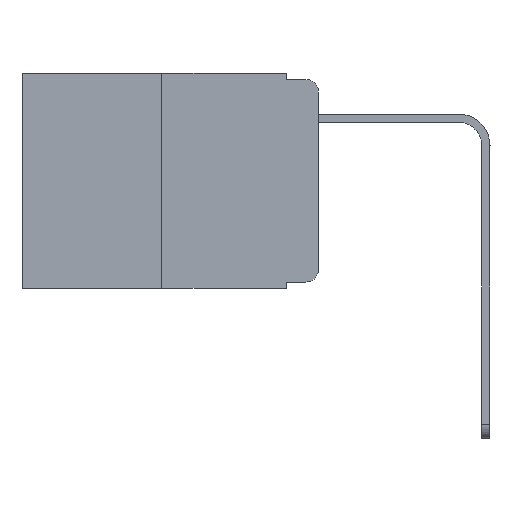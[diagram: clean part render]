
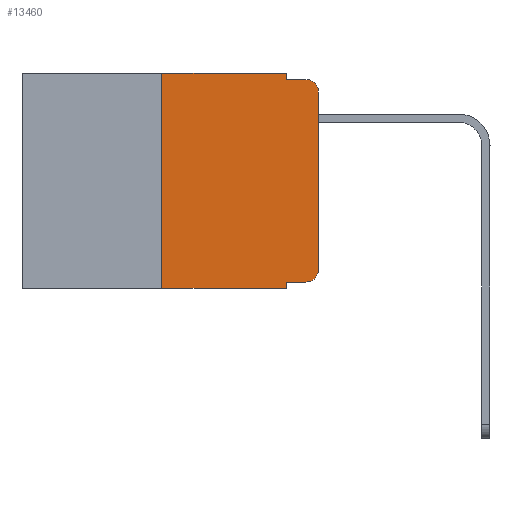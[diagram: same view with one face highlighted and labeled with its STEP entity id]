
A CAD part, left-side view. The second image highlights one B-rep face of the part: STEP entity #13460.
In plain terms, the highlighted planar face has unit normal (-1, 0, 0).
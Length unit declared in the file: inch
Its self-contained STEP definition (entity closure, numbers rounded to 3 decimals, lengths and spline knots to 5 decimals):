
#66 = ORIENTED_EDGE ( 'NONE', *, *, #15885, .T. ) ;
#69 = DIRECTION ( 'NONE',  ( 0., 0., -1. ) ) ;
#484 = CARTESIAN_POINT ( 'NONE',  ( 0., 0.051, -0.333 ) ) ;
#685 = CARTESIAN_POINT ( 'NONE',  ( 0., 0.02, -0.313 ) ) ;
#712 = CARTESIAN_POINT ( 'NONE',  ( 0., 0.473, 0. ) ) ;
#753 = VERTEX_POINT ( 'NONE', #1145 ) ;
#788 = CARTESIAN_POINT ( 'NONE',  ( 0., 0.02, -0.333 ) ) ;
#983 = AXIS2_PLACEMENT_3D ( 'NONE', #712, #11700, #2140 ) ;
#1099 = VERTEX_POINT ( 'NONE', #9151 ) ;
#1145 = CARTESIAN_POINT ( 'NONE',  ( 0., 0.051, 0. ) ) ;
#1576 = CARTESIAN_POINT ( 'NONE',  ( 0., 0.25, 0. ) ) ;
#1659 = CARTESIAN_POINT ( 'NONE',  ( 0., 0., -0.313 ) ) ;
#1747 = CARTESIAN_POINT ( 'NONE',  ( 0., 0.051, -0.01 ) ) ;
#1787 = CARTESIAN_POINT ( 'NONE',  ( 0., 0.473, -0.343 ) ) ;
#2140 = DIRECTION ( 'NONE',  ( 0., 0., -1. ) ) ;
#2186 = AXIS2_PLACEMENT_3D ( 'NONE', #685, #13418, #4994 ) ;
#2284 = ORIENTED_EDGE ( 'NONE', *, *, #7807, .F. ) ;
#2453 = VERTEX_POINT ( 'NONE', #1747 ) ;
#2645 = ORIENTED_EDGE ( 'NONE', *, *, #8394, .T. ) ;
#2680 = EDGE_CURVE ( 'NONE', #7427, #15474, #4376, .T. ) ;
#2983 = FACE_OUTER_BOUND ( 'NONE', #12469, .T. ) ;
#3580 = LINE ( 'NONE', #10822, #18109 ) ;
#3884 = CARTESIAN_POINT ( 'NONE',  ( 0., 0.051, -0.01 ) ) ;
#3978 = VERTEX_POINT ( 'NONE', #9207 ) ;
#4061 = CARTESIAN_POINT ( 'NONE',  ( 0., 0.02, -0.01 ) ) ;
#4107 = VECTOR ( 'NONE', #14546, 39.37008 ) ;
#4376 = CIRCLE ( 'NONE', #2186, 0.02 ) ;
#4994 = DIRECTION ( 'NONE',  ( 0., 0., -1. ) ) ;
#5096 = EDGE_CURVE ( 'NONE', #13319, #7427, #9376, .T. ) ;
#5805 = CARTESIAN_POINT ( 'NONE',  ( 0., 0.051, -0.333 ) ) ;
#6109 = EDGE_CURVE ( 'NONE', #753, #2453, #14809, .T. ) ;
#6309 = ORIENTED_EDGE ( 'NONE', *, *, #13696, .T. ) ;
#6413 = VERTEX_POINT ( 'NONE', #13364 ) ;
#6456 = ORIENTED_EDGE ( 'NONE', *, *, #7017, .F. ) ;
#6510 = CARTESIAN_POINT ( 'NONE',  ( 0., 0.02, -0.03 ) ) ;
#7017 = EDGE_CURVE ( 'NONE', #2453, #7630, #15676, .T. ) ;
#7042 = EDGE_CURVE ( 'NONE', #3978, #753, #3580, .T. ) ;
#7072 = CARTESIAN_POINT ( 'NONE',  ( 0., 0.051, 0. ) ) ;
#7427 = VERTEX_POINT ( 'NONE', #788 ) ;
#7570 = VECTOR ( 'NONE', #11715, 39.37008 ) ;
#7630 = VERTEX_POINT ( 'NONE', #4061 ) ;
#7807 = EDGE_CURVE ( 'NONE', #1099, #3978, #15631, .T. ) ;
#7933 = DIRECTION ( 'NONE',  ( 0., 0., -1. ) ) ;
#8123 = DIRECTION ( 'NONE',  ( 0., -1., 0. ) ) ;
#8161 = CARTESIAN_POINT ( 'NONE',  ( 0., 0., 0. ) ) ;
#8382 = VECTOR ( 'NONE', #17199, 39.37008 ) ;
#8394 = EDGE_CURVE ( 'NONE', #1099, #17314, #15501, .T. ) ;
#8700 = VECTOR ( 'NONE', #13808, 39.37008 ) ;
#9151 = CARTESIAN_POINT ( 'NONE',  ( 0., 0.25, -0.343 ) ) ;
#9207 = CARTESIAN_POINT ( 'NONE',  ( 0., 0.25, 0. ) ) ;
#9376 = LINE ( 'NONE', #484, #4107 ) ;
#9874 = CIRCLE ( 'NONE', #17280, 0.02 ) ;
#10047 = LINE ( 'NONE', #7072, #16225 ) ;
#10822 = CARTESIAN_POINT ( 'NONE',  ( 0., 0.473, 0. ) ) ;
#11552 = DIRECTION ( 'NONE',  ( 0., -1., 0. ) ) ;
#11700 = DIRECTION ( 'NONE',  ( 1., 0., 0. ) ) ;
#11715 = DIRECTION ( 'NONE',  ( 0., 0., -1. ) ) ;
#11766 = PLANE ( 'NONE',  #983 ) ;
#11778 = LINE ( 'NONE', #8161, #8700 ) ;
#11846 = CARTESIAN_POINT ( 'NONE',  ( 0., 0.051, 0. ) ) ;
#11931 = VECTOR ( 'NONE', #12100, 39.37008 ) ;
#12100 = DIRECTION ( 'NONE',  ( 0., -1., 0. ) ) ;
#12201 = CARTESIAN_POINT ( 'NONE',  ( 0., 0.051, -0.343 ) ) ;
#12261 = ORIENTED_EDGE ( 'NONE', *, *, #5096, .T. ) ;
#12469 = EDGE_LOOP ( 'NONE', ( #6309, #66, #6456, #13913, #17244, #2284, #2645, #12553, #12261, #15626 ) ) ;
#12492 = EDGE_CURVE ( 'NONE', #13319, #17314, #10047, .T. ) ;
#12553 = ORIENTED_EDGE ( 'NONE', *, *, #12492, .F. ) ;
#13319 = VERTEX_POINT ( 'NONE', #5805 ) ;
#13364 = CARTESIAN_POINT ( 'NONE',  ( 0., 0., -0.03 ) ) ;
#13418 = DIRECTION ( 'NONE',  ( -1., 0., 0. ) ) ;
#13460 = ADVANCED_FACE ( 'NONE', ( #2983 ), #11766, .F. ) ;
#13696 = EDGE_CURVE ( 'NONE', #15474, #6413, #11778, .T. ) ;
#13808 = DIRECTION ( 'NONE',  ( 0., 0., 1. ) ) ;
#13913 = ORIENTED_EDGE ( 'NONE', *, *, #6109, .F. ) ;
#14546 = DIRECTION ( 'NONE',  ( 0., -1., 0. ) ) ;
#14809 = LINE ( 'NONE', #11846, #7570 ) ;
#15474 = VERTEX_POINT ( 'NONE', #1659 ) ;
#15501 = LINE ( 'NONE', #1787, #16831 ) ;
#15626 = ORIENTED_EDGE ( 'NONE', *, *, #2680, .T. ) ;
#15631 = LINE ( 'NONE', #1576, #8382 ) ;
#15676 = LINE ( 'NONE', #3884, #11931 ) ;
#15885 = EDGE_CURVE ( 'NONE', #6413, #7630, #9874, .T. ) ;
#16225 = VECTOR ( 'NONE', #69, 39.37008 ) ;
#16350 = DIRECTION ( 'NONE',  ( -1., 0., 0. ) ) ;
#16831 = VECTOR ( 'NONE', #11552, 39.37008 ) ;
#17199 = DIRECTION ( 'NONE',  ( 0., 0., 1. ) ) ;
#17244 = ORIENTED_EDGE ( 'NONE', *, *, #7042, .F. ) ;
#17280 = AXIS2_PLACEMENT_3D ( 'NONE', #6510, #16350, #7933 ) ;
#17314 = VERTEX_POINT ( 'NONE', #12201 ) ;
#18109 = VECTOR ( 'NONE', #8123, 39.37008 ) ;
